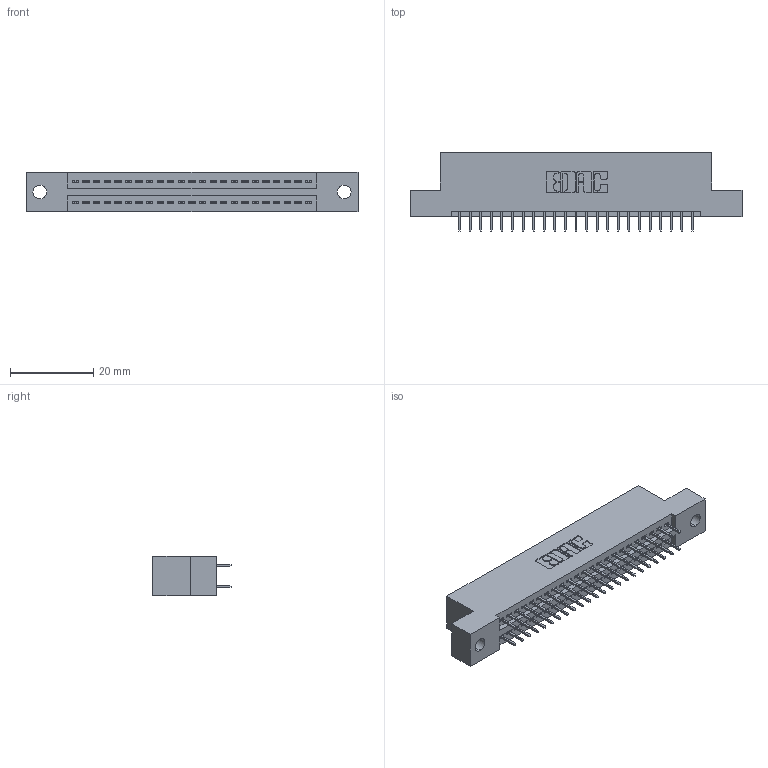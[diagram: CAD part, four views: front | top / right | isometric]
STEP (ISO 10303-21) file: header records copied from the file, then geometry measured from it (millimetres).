
FILE_DESCRIPTION (( 'STEP AP203' ), '1' );
FILE_NAME ('895-046-525-202.STEP', '2020-09-27T05:18:54', ( '' ), ( '' ), 'SwSTEP 2.0', 'SolidWorks 2020', '' );
FILE_SCHEMA (( 'CONFIG_CONTROL_DESIGN' ));
Length unit declared in the file: inch
Products named in the file (3): 845 Part_Flush Mounting Lugs - 0.128 Dia; 345-292-001_345-293-125; 895-046-525-202
Assembly tree (47 placements, depth 2):
  895-046-525-202
    845 Part_Flush Mounting Lugs - 0.128 Dia
    345-292-001_345-293-125  x46
Bounding box: 79.63 x 18.72 x 9.4 mm (x, y, z)
Volume: 7446.5 mm3; surface area: 10138.3 mm2
Topology: 47 solids, 47 shells, 2610 faces, 7379 edges, 4734 vertices
Faces by surface type: plane 1874, cylinder 736
Entity records: 20681 total; most frequent: CARTESIAN_POINT 3484, ORIENTED_EDGE 3418, DIRECTION 3097, EDGE_CURVE 1709, VECTOR 1489, LINE 1489, VERTEX_POINT 1134, AXIS2_PLACEMENT_3D 804
